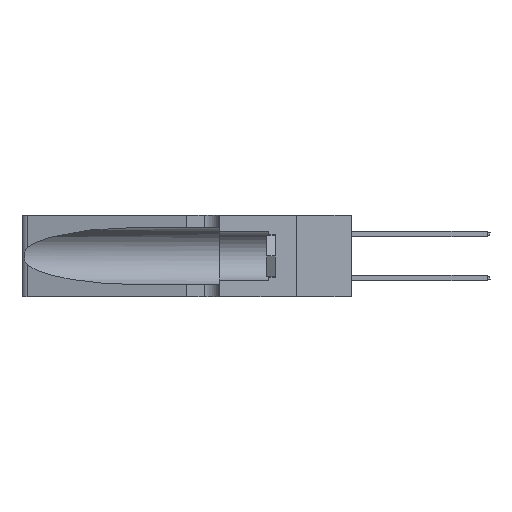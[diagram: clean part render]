
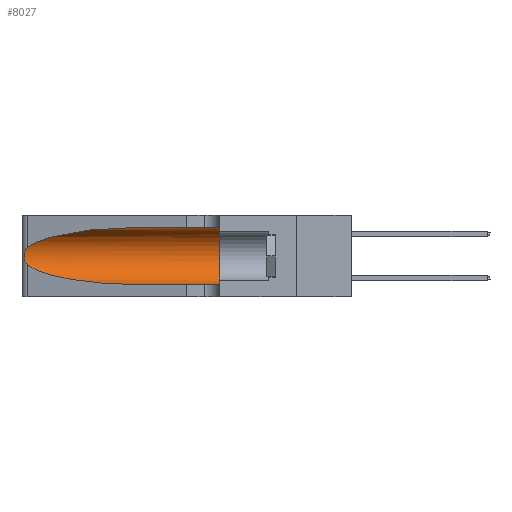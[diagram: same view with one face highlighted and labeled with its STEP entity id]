
A CAD part, left-side view. The second image highlights one B-rep face of the part: STEP entity #8027.
In plain terms, the highlighted cylindrical face has radius 3.308 mm (diameter 6.617 mm), a partial arc.
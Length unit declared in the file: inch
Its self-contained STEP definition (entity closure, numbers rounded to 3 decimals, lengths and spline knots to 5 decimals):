
#290 = CARTESIAN_POINT ( 'NONE',  ( 0.1305, 0.35, 0.05475 ) ) ;
#1366 =( BOUNDED_CURVE ( )  B_SPLINE_CURVE ( 3, ( #5181, #9215, #31808, #35549 ),
 .UNSPECIFIED., .F., .F. ) 
 B_SPLINE_CURVE_WITH_KNOTS ( ( 4, 4 ),
 ( 1.5708, 2.84003 ),
 .UNSPECIFIED. ) 
 CURVE ( )  GEOMETRIC_REPRESENTATION_ITEM ( )  RATIONAL_B_SPLINE_CURVE ( ( 1., 0.87, 0.87, 1. ) ) 
 REPRESENTATION_ITEM ( '' )  );
#2404 = EDGE_CURVE ( 'NONE', #42427, #27983, #1366, .T. ) ;
#2880 = CARTESIAN_POINT ( 'NONE',  ( 0.1305, 1.61858, 0.31525 ) ) ;
#2994 = CARTESIAN_POINT ( 'NONE',  ( 0.25789, 1.23486, 0.15765 ) ) ;
#5082 = CARTESIAN_POINT ( 'NONE',  ( 0.1305, 0.72297, 0.05475 ) ) ;
#5181 = CARTESIAN_POINT ( 'NONE',  ( 0.1305, 0.72297, 0.31525 ) ) ;
#5665 = CYLINDRICAL_SURFACE ( 'NONE', #48081, 0.13025 ) ;
#6726 = CARTESIAN_POINT ( 'NONE',  ( 0.25487, 1.22718, 0.22369 ) ) ;
#6891 = CARTESIAN_POINT ( 'NONE',  ( 0.25555, 1.22993, 0.14849 ) ) ;
#8027 = ADVANCED_FACE ( 'NONE', ( #35777 ), #5665, .F. ) ;
#8065 = EDGE_CURVE ( 'NONE', #11566, #37409, #33000, .T. ) ;
#9215 = CARTESIAN_POINT ( 'NONE',  ( 0.18966, 0.96281, 0.31525 ) ) ;
#11068 = CARTESIAN_POINT ( 'NONE',  ( 0.25487, 1.22718, 0.22369 ) ) ;
#11566 = VERTEX_POINT ( 'NONE', #37758 ) ;
#12593 = CARTESIAN_POINT ( 'NONE',  ( 0.1305, 0.35, 0.185 ) ) ;
#14092 = EDGE_LOOP ( 'NONE', ( #14832, #18380, #48169, #41767, #35444, #26672 ) ) ;
#14348 = CARTESIAN_POINT ( 'NONE',  ( 0.25787, 1.23484, 0.2124 ) ) ;
#14478 = VECTOR ( 'NONE', #34808, 39.37008 ) ;
#14832 = ORIENTED_EDGE ( 'NONE', *, *, #2404, .T. ) ;
#15668 = LINE ( 'NONE', #27448, #14478 ) ;
#16405 = DIRECTION ( 'NONE',  ( 0., 0., 1. ) ) ;
#17654 = CARTESIAN_POINT ( 'NONE',  ( 0.18966, 0.96281, 0.05475 ) ) ;
#18140 = CARTESIAN_POINT ( 'NONE',  ( 0.26018, 1.23835, 0.19895 ) ) ;
#18380 = ORIENTED_EDGE ( 'NONE', *, *, #28859, .T. ) ;
#18616 = CIRCLE ( 'NONE', #44236, 0.13025 ) ;
#20387 = EDGE_CURVE ( 'NONE', #37409, #46704, #15668, .T. ) ;
#21155 = CARTESIAN_POINT ( 'NONE',  ( 0.1305, 1.61858, 0.185 ) ) ;
#21970 = CARTESIAN_POINT ( 'NONE',  ( 0.26075, 1.23896, 0.178 ) ) ;
#23518 = VECTOR ( 'NONE', #25604, 39.37008 ) ;
#24919 = DIRECTION ( 'NONE',  ( 0., -1., 0. ) ) ;
#25604 = DIRECTION ( 'NONE',  ( 0., -1., 0. ) ) ;
#25724 = CARTESIAN_POINT ( 'NONE',  ( 0.25856, 1.23593, 0.16098 ) ) ;
#26672 = ORIENTED_EDGE ( 'NONE', *, *, #42869, .F. ) ;
#27448 = CARTESIAN_POINT ( 'NONE',  ( 0.1305, 1.61858, 0.05475 ) ) ;
#27983 = VERTEX_POINT ( 'NONE', #11068 ) ;
#28859 = EDGE_CURVE ( 'NONE', #27983, #11566, #38055, .T. ) ;
#29499 = CARTESIAN_POINT ( 'NONE',  ( 0.25639, 1.23186, 0.15144 ) ) ;
#31808 = CARTESIAN_POINT ( 'NONE',  ( 0.2373, 1.15595, 0.28018 ) ) ;
#32315 = LINE ( 'NONE', #2880, #23518 ) ;
#32480 = CARTESIAN_POINT ( 'NONE',  ( 0.1305, 0.35, 0.31525 ) ) ;
#33000 =( BOUNDED_CURVE ( )  B_SPLINE_CURVE ( 3, ( #43783, #36383, #17654, #47544 ),
 .UNSPECIFIED., .F., .F. ) 
 B_SPLINE_CURVE_WITH_KNOTS ( ( 4, 4 ),
 ( 3.44316, 4.71239 ),
 .UNSPECIFIED. ) 
 CURVE ( )  GEOMETRIC_REPRESENTATION_ITEM ( )  RATIONAL_B_SPLINE_CURVE ( ( 1., 0.87, 0.87, 1. ) ) 
 REPRESENTATION_ITEM ( '' )  );
#33125 = CARTESIAN_POINT ( 'NONE',  ( 0.25555, 1.22994, 0.2215 ) ) ;
#33297 = CARTESIAN_POINT ( 'NONE',  ( 0.25487, 1.22718, 0.14631 ) ) ;
#34176 = VERTEX_POINT ( 'NONE', #32480 ) ;
#34808 = DIRECTION ( 'NONE',  ( 0., -1., 0. ) ) ;
#35444 = ORIENTED_EDGE ( 'NONE', *, *, #39222, .F. ) ;
#35549 = CARTESIAN_POINT ( 'NONE',  ( 0.25487, 1.22718, 0.22369 ) ) ;
#35777 = FACE_OUTER_BOUND ( 'NONE', #14092, .T. ) ;
#36383 = CARTESIAN_POINT ( 'NONE',  ( 0.2373, 1.15595, 0.08982 ) ) ;
#36870 = CARTESIAN_POINT ( 'NONE',  ( 0.25639, 1.23184, 0.21858 ) ) ;
#37409 = VERTEX_POINT ( 'NONE', #5082 ) ;
#37758 = CARTESIAN_POINT ( 'NONE',  ( 0.25487, 1.22718, 0.14631 ) ) ;
#38055 = B_SPLINE_CURVE_WITH_KNOTS ( 'NONE', 3,
 ( #6726, #33125, #36870, #14348, #40560, #18140, #44281, #21970, #48021, #25724, #2994, #29499, #6891, #33297 ),
 .UNSPECIFIED., .F., .F.,
 ( 4, 2, 2, 2, 2, 2, 4 ),
 ( 0., 0.00027, 0.00053, 0.00107, 0.0016, 0.00187, 0.00214 ),
 .UNSPECIFIED. ) ;
#38861 = DIRECTION ( 'NONE',  ( 0., 1., 0. ) ) ;
#39222 = EDGE_CURVE ( 'NONE', #34176, #46704, #18616, .T. ) ;
#40560 = CARTESIAN_POINT ( 'NONE',  ( 0.25854, 1.2359, 0.20912 ) ) ;
#40952 = CARTESIAN_POINT ( 'NONE',  ( 0.1305, 0.72297, 0.31525 ) ) ;
#41767 = ORIENTED_EDGE ( 'NONE', *, *, #20387, .T. ) ;
#42427 = VERTEX_POINT ( 'NONE', #40952 ) ;
#42869 = EDGE_CURVE ( 'NONE', #42427, #34176, #32315, .T. ) ;
#43466 = DIRECTION ( 'NONE',  ( 0., 0., -1. ) ) ;
#43783 = CARTESIAN_POINT ( 'NONE',  ( 0.25487, 1.22718, 0.14631 ) ) ;
#44236 = AXIS2_PLACEMENT_3D ( 'NONE', #12593, #38861, #16405 ) ;
#44281 = CARTESIAN_POINT ( 'NONE',  ( 0.26075, 1.23896, 0.19203 ) ) ;
#46704 = VERTEX_POINT ( 'NONE', #290 ) ;
#47544 = CARTESIAN_POINT ( 'NONE',  ( 0.1305, 0.72297, 0.05475 ) ) ;
#48021 = CARTESIAN_POINT ( 'NONE',  ( 0.26017, 1.23833, 0.17102 ) ) ;
#48081 = AXIS2_PLACEMENT_3D ( 'NONE', #21155, #24919, #43466 ) ;
#48169 = ORIENTED_EDGE ( 'NONE', *, *, #8065, .T. ) ;
